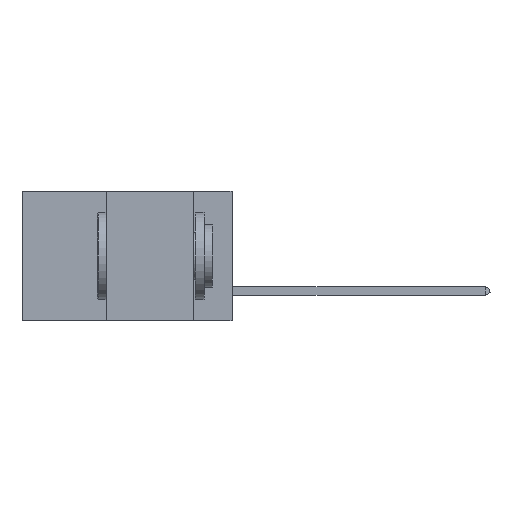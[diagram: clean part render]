
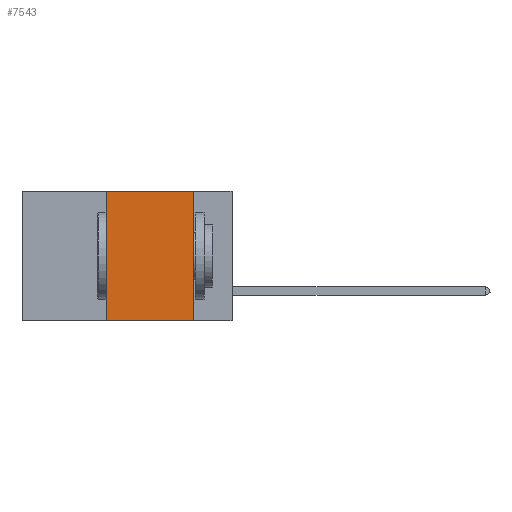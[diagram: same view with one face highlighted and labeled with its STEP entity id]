
A CAD part, left-side view. The second image highlights one B-rep face of the part: STEP entity #7543.
In plain terms, the highlighted planar face has unit normal (-1, 0, 0).
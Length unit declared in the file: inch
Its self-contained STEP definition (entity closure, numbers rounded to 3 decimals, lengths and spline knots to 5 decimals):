
#90 = AXIS2_PLACEMENT_3D ( 'NONE', #10039, #18671, #8465 ) ;
#223 = PLANE ( 'NONE',  #90 ) ;
#437 = VECTOR ( 'NONE', #11052, 39.37008 ) ;
#539 = CARTESIAN_POINT ( 'NONE',  ( 0., 0.11, 0. ) ) ;
#1951 = LINE ( 'NONE', #539, #9613 ) ;
#2291 = DIRECTION ( 'NONE',  ( 0., 0., -1. ) ) ;
#2510 = CARTESIAN_POINT ( 'NONE',  ( 0., 0.11, 0. ) ) ;
#2745 = ORIENTED_EDGE ( 'NONE', *, *, #5993, .F. ) ;
#3886 = ORIENTED_EDGE ( 'NONE', *, *, #18010, .F. ) ;
#4091 = ORIENTED_EDGE ( 'NONE', *, *, #14792, .F. ) ;
#5970 = CARTESIAN_POINT ( 'NONE',  ( 0., 0.36, -0.37 ) ) ;
#5993 = EDGE_CURVE ( 'NONE', #18112, #7176, #1951, .T. ) ;
#7176 = VERTEX_POINT ( 'NONE', #17763 ) ;
#7543 = ADVANCED_FACE ( 'NONE', ( #19653 ), #223, .F. ) ;
#7674 = CARTESIAN_POINT ( 'NONE',  ( 0., 0.36, 0. ) ) ;
#8465 = DIRECTION ( 'NONE',  ( 0., 0., -1. ) ) ;
#9613 = VECTOR ( 'NONE', #2291, 39.37008 ) ;
#10039 = CARTESIAN_POINT ( 'NONE',  ( 0., 0.6, 0. ) ) ;
#10440 = LINE ( 'NONE', #7674, #437 ) ;
#10583 = CARTESIAN_POINT ( 'NONE',  ( 0., 0.36, 0. ) ) ;
#11052 = DIRECTION ( 'NONE',  ( 0., 0., 1. ) ) ;
#11378 = EDGE_CURVE ( 'NONE', #21304, #7176, #17587, .T. ) ;
#13018 = VECTOR ( 'NONE', #13994, 39.37008 ) ;
#13765 = CARTESIAN_POINT ( 'NONE',  ( 0., 0.6, -0.37 ) ) ;
#13994 = DIRECTION ( 'NONE',  ( 0., -1., 0. ) ) ;
#14792 = EDGE_CURVE ( 'NONE', #21304, #16539, #10440, .T. ) ;
#15146 = ORIENTED_EDGE ( 'NONE', *, *, #11378, .T. ) ;
#15317 = CARTESIAN_POINT ( 'NONE',  ( 0., 0.6, 0. ) ) ;
#15474 = DIRECTION ( 'NONE',  ( 0., -1., 0. ) ) ;
#16174 = LINE ( 'NONE', #15317, #18573 ) ;
#16525 = EDGE_LOOP ( 'NONE', ( #2745, #3886, #4091, #15146 ) ) ;
#16539 = VERTEX_POINT ( 'NONE', #10583 ) ;
#17587 = LINE ( 'NONE', #13765, #13018 ) ;
#17763 = CARTESIAN_POINT ( 'NONE',  ( 0., 0.11, -0.37 ) ) ;
#18010 = EDGE_CURVE ( 'NONE', #16539, #18112, #16174, .T. ) ;
#18112 = VERTEX_POINT ( 'NONE', #2510 ) ;
#18573 = VECTOR ( 'NONE', #15474, 39.37008 ) ;
#18671 = DIRECTION ( 'NONE',  ( 1., 0., 0. ) ) ;
#19653 = FACE_OUTER_BOUND ( 'NONE', #16525, .T. ) ;
#21304 = VERTEX_POINT ( 'NONE', #5970 ) ;
